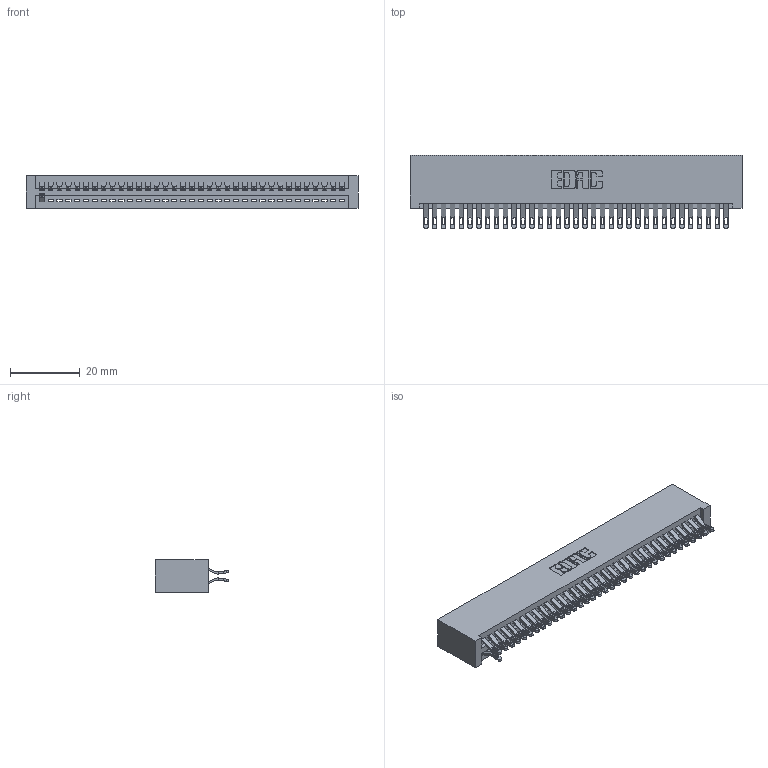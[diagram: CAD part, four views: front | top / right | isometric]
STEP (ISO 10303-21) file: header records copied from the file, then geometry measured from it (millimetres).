
FILE_DESCRIPTION (( 'STEP AP203' ), '1' );
FILE_NAME ('395-070-555-201.STEP', '2018-11-27T00:00:10', ( '' ), ( '' ), 'SwSTEP 2.0', 'SolidWorks 2016', '' );
FILE_SCHEMA (( 'CONFIG_CONTROL_DESIGN' ));
Length unit declared in the file: inch
Products named in the file (3): 345 Part_No Mounting Lugs; 345-292-001_555 Tail; 395-070-555-201
Assembly tree (37 placements, depth 2):
  395-070-555-201
    345 Part_No Mounting Lugs
    345-292-001_555 Tail  x36
Bounding box: 95.5 x 21.13 x 9.4 mm (x, y, z)
Volume: 9626.2 mm3; surface area: 13024.2 mm2
Topology: 37 solids, 37 shells, 2406 faces, 7607 edges, 5070 vertices
Faces by surface type: plane 1430, cylinder 976
Entity records: 27365 total; most frequent: CARTESIAN_POINT 4776, ORIENTED_EDGE 4714, DIRECTION 4145, EDGE_CURVE 2357, LINE 2073, VECTOR 2073, VERTEX_POINT 1570, AXIS2_PLACEMENT_3D 1036
